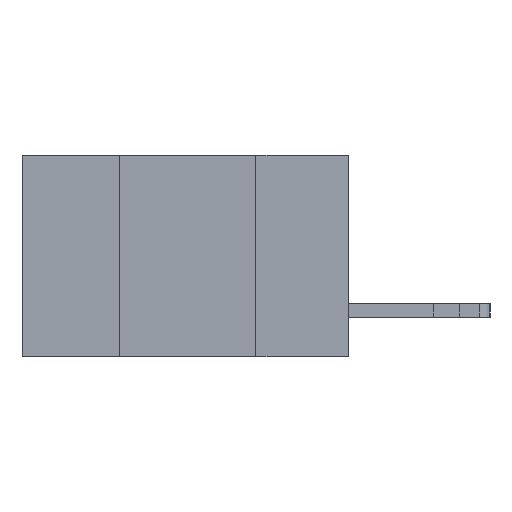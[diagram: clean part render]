
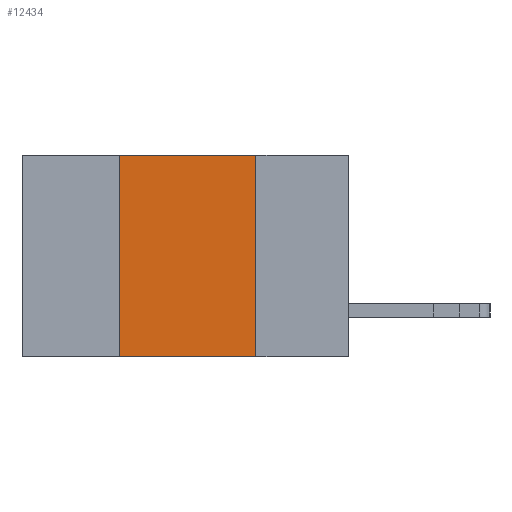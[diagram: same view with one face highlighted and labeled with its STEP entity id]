
A CAD part, left-side view. The second image highlights one B-rep face of the part: STEP entity #12434.
In plain terms, the highlighted planar face has unit normal (-1, 0, 0).
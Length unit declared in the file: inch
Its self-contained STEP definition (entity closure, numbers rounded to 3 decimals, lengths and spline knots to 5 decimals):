
#335 = EDGE_CURVE ( 'NONE', #5913, #13959, #24144, .T. ) ;
#350 = CARTESIAN_POINT ( 'NONE',  ( 0., 0.42, -0.37 ) ) ;
#772 = VECTOR ( 'NONE', #2390, 39.37008 ) ;
#1144 = VECTOR ( 'NONE', #15723, 39.37008 ) ;
#2390 = DIRECTION ( 'NONE',  ( 0., 0., 1. ) ) ;
#2426 = LINE ( 'NONE', #9567, #1144 ) ;
#2598 = VECTOR ( 'NONE', #4627, 39.37008 ) ;
#4602 = VERTEX_POINT ( 'NONE', #5933 ) ;
#4627 = DIRECTION ( 'NONE',  ( 0., -1., 0. ) ) ;
#5913 = VERTEX_POINT ( 'NONE', #8917 ) ;
#5933 = CARTESIAN_POINT ( 'NONE',  ( 0., 0.42, -0.37 ) ) ;
#6118 = ORIENTED_EDGE ( 'NONE', *, *, #7318, .T. ) ;
#6773 = ORIENTED_EDGE ( 'NONE', *, *, #335, .F. ) ;
#7199 = CARTESIAN_POINT ( 'NONE',  ( 0., 0.17, -0.37 ) ) ;
#7318 = EDGE_CURVE ( 'NONE', #4602, #20586, #2426, .T. ) ;
#7417 = ORIENTED_EDGE ( 'NONE', *, *, #11042, .F. ) ;
#8537 = PLANE ( 'NONE',  #21241 ) ;
#8604 = CARTESIAN_POINT ( 'NONE',  ( 0., 0.17, -0.37 ) ) ;
#8917 = CARTESIAN_POINT ( 'NONE',  ( 0., 0.42, 0. ) ) ;
#9567 = CARTESIAN_POINT ( 'NONE',  ( 0., 0.6, -0.37 ) ) ;
#9631 = VECTOR ( 'NONE', #22740, 39.37008 ) ;
#10587 = DIRECTION ( 'NONE',  ( 0., 0., -1. ) ) ;
#11042 = EDGE_CURVE ( 'NONE', #13959, #20586, #13160, .T. ) ;
#11634 = LINE ( 'NONE', #350, #772 ) ;
#12434 = ADVANCED_FACE ( 'NONE', ( #17175 ), #8537, .F. ) ;
#13160 = LINE ( 'NONE', #8604, #9631 ) ;
#13418 = EDGE_LOOP ( 'NONE', ( #7417, #6773, #22289, #6118 ) ) ;
#13959 = VERTEX_POINT ( 'NONE', #16551 ) ;
#15259 = CARTESIAN_POINT ( 'NONE',  ( 0., 0.6, 0. ) ) ;
#15723 = DIRECTION ( 'NONE',  ( 0., -1., 0. ) ) ;
#16551 = CARTESIAN_POINT ( 'NONE',  ( 0., 0.17, 0. ) ) ;
#17175 = FACE_OUTER_BOUND ( 'NONE', #13418, .T. ) ;
#18094 = EDGE_CURVE ( 'NONE', #4602, #5913, #11634, .T. ) ;
#20577 = CARTESIAN_POINT ( 'NONE',  ( 0., 0.6, 0. ) ) ;
#20586 = VERTEX_POINT ( 'NONE', #7199 ) ;
#21241 = AXIS2_PLACEMENT_3D ( 'NONE', #20577, #22685, #10587 ) ;
#22289 = ORIENTED_EDGE ( 'NONE', *, *, #18094, .F. ) ;
#22685 = DIRECTION ( 'NONE',  ( 1., 0., 0. ) ) ;
#22740 = DIRECTION ( 'NONE',  ( 0., 0., -1. ) ) ;
#24144 = LINE ( 'NONE', #15259, #2598 ) ;
